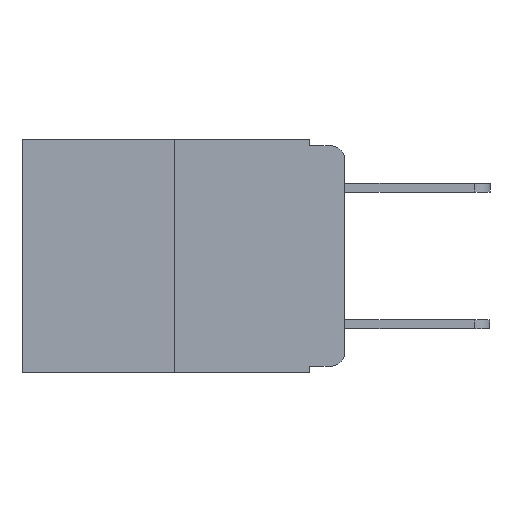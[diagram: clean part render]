
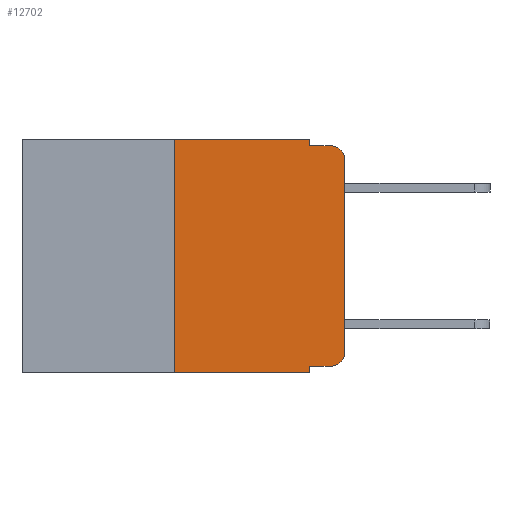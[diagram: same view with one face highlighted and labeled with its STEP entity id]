
A CAD part, left-side view. The second image highlights one B-rep face of the part: STEP entity #12702.
In plain terms, the highlighted planar face has unit normal (-1, 0, 0).
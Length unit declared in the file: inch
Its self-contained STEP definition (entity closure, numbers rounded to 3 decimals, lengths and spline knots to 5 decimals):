
#7 = CARTESIAN_POINT ( 'NONE',  ( 0., 0.051, -0.333 ) ) ;
#432 = DIRECTION ( 'NONE',  ( 0., 0., -1. ) ) ;
#626 = CARTESIAN_POINT ( 'NONE',  ( 0., 0.25, 0. ) ) ;
#860 = DIRECTION ( 'NONE',  ( 0., 0., -1. ) ) ;
#1027 = EDGE_CURVE ( 'NONE', #7281, #16380, #20398, .T. ) ;
#2823 = CARTESIAN_POINT ( 'NONE',  ( 0., 0.25, 0. ) ) ;
#3189 = VECTOR ( 'NONE', #7980, 39.37008 ) ;
#3212 = CARTESIAN_POINT ( 'NONE',  ( 0., 0., 0. ) ) ;
#3358 = ORIENTED_EDGE ( 'NONE', *, *, #3639, .T. ) ;
#3364 = CARTESIAN_POINT ( 'NONE',  ( 0., 0.051, -0.333 ) ) ;
#3558 = VERTEX_POINT ( 'NONE', #4298 ) ;
#3639 = EDGE_CURVE ( 'NONE', #3558, #7281, #15015, .T. ) ;
#3943 = EDGE_CURVE ( 'NONE', #13110, #13156, #8935, .T. ) ;
#4298 = CARTESIAN_POINT ( 'NONE',  ( 0., 0.02, -0.333 ) ) ;
#4719 = CARTESIAN_POINT ( 'NONE',  ( 0., 0.473, 0. ) ) ;
#4754 = AXIS2_PLACEMENT_3D ( 'NONE', #20390, #20478, #11328 ) ;
#5233 = ORIENTED_EDGE ( 'NONE', *, *, #3943, .F. ) ;
#5365 = DIRECTION ( 'NONE',  ( -1., 0., 0. ) ) ;
#5609 = PLANE ( 'NONE',  #8945 ) ;
#6151 = DIRECTION ( 'NONE',  ( 0., 0., 1. ) ) ;
#6529 = AXIS2_PLACEMENT_3D ( 'NONE', #15492, #5365, #17217 ) ;
#6669 = EDGE_CURVE ( 'NONE', #13178, #18244, #18235, .T. ) ;
#6810 = VECTOR ( 'NONE', #10168, 39.37008 ) ;
#7281 = VERTEX_POINT ( 'NONE', #12717 ) ;
#7354 = LINE ( 'NONE', #3364, #6810 ) ;
#7600 = ORIENTED_EDGE ( 'NONE', *, *, #8977, .F. ) ;
#7980 = DIRECTION ( 'NONE',  ( 0., -1., 0. ) ) ;
#8057 = VERTEX_POINT ( 'NONE', #10492 ) ;
#8070 = VECTOR ( 'NONE', #15999, 39.37008 ) ;
#8119 = DIRECTION ( 'NONE',  ( 0., -1., 0. ) ) ;
#8129 = VERTEX_POINT ( 'NONE', #19088 ) ;
#8935 = LINE ( 'NONE', #10293, #21849 ) ;
#8945 = AXIS2_PLACEMENT_3D ( 'NONE', #20779, #10669, #432 ) ;
#8977 = EDGE_CURVE ( 'NONE', #17702, #13110, #15774, .T. ) ;
#9217 = VECTOR ( 'NONE', #11087, 39.37008 ) ;
#9340 = CARTESIAN_POINT ( 'NONE',  ( 0., 0.051, -0.343 ) ) ;
#9372 = CARTESIAN_POINT ( 'NONE',  ( 0., 0.051, 0. ) ) ;
#9766 = ORIENTED_EDGE ( 'NONE', *, *, #1027, .T. ) ;
#9867 = DIRECTION ( 'NONE',  ( 0., -1., 0. ) ) ;
#10036 = EDGE_CURVE ( 'NONE', #8129, #17702, #12577, .T. ) ;
#10057 = CARTESIAN_POINT ( 'NONE',  ( 0., 0.051, 0. ) ) ;
#10168 = DIRECTION ( 'NONE',  ( 0., -1., 0. ) ) ;
#10293 = CARTESIAN_POINT ( 'NONE',  ( 0., 0.051, 0. ) ) ;
#10492 = CARTESIAN_POINT ( 'NONE',  ( 0., 0.02, -0.01 ) ) ;
#10669 = DIRECTION ( 'NONE',  ( 1., 0., 0. ) ) ;
#11087 = DIRECTION ( 'NONE',  ( 0., 0., -1. ) ) ;
#11268 = VECTOR ( 'NONE', #8119, 39.37008 ) ;
#11328 = DIRECTION ( 'NONE',  ( 0., 0., -1. ) ) ;
#12577 = LINE ( 'NONE', #626, #8070 ) ;
#12702 = ADVANCED_FACE ( 'NONE', ( #13420 ), #5609, .F. ) ;
#12717 = CARTESIAN_POINT ( 'NONE',  ( 0., 0., -0.313 ) ) ;
#13110 = VERTEX_POINT ( 'NONE', #10057 ) ;
#13156 = VERTEX_POINT ( 'NONE', #21993 ) ;
#13178 = VERTEX_POINT ( 'NONE', #7 ) ;
#13420 = FACE_OUTER_BOUND ( 'NONE', #16787, .T. ) ;
#14911 = CARTESIAN_POINT ( 'NONE',  ( 0., 0.473, -0.343 ) ) ;
#15015 = CIRCLE ( 'NONE', #4754, 0.02 ) ;
#15040 = ORIENTED_EDGE ( 'NONE', *, *, #20939, .F. ) ;
#15492 = CARTESIAN_POINT ( 'NONE',  ( 0., 0.02, -0.03 ) ) ;
#15774 = LINE ( 'NONE', #4719, #11268 ) ;
#15941 = ORIENTED_EDGE ( 'NONE', *, *, #21018, .T. ) ;
#15999 = DIRECTION ( 'NONE',  ( 0., 0., 1. ) ) ;
#16123 = ORIENTED_EDGE ( 'NONE', *, *, #6669, .F. ) ;
#16374 = ORIENTED_EDGE ( 'NONE', *, *, #10036, .F. ) ;
#16380 = VERTEX_POINT ( 'NONE', #20914 ) ;
#16411 = CARTESIAN_POINT ( 'NONE',  ( 0., 0.051, -0.01 ) ) ;
#16787 = EDGE_LOOP ( 'NONE', ( #9766, #18763, #15040, #5233, #7600, #16374, #15941, #16123, #17990, #3358 ) ) ;
#17217 = DIRECTION ( 'NONE',  ( 0., 0., -1. ) ) ;
#17312 = EDGE_CURVE ( 'NONE', #13178, #3558, #7354, .T. ) ;
#17702 = VERTEX_POINT ( 'NONE', #2823 ) ;
#17990 = ORIENTED_EDGE ( 'NONE', *, *, #17312, .T. ) ;
#18235 = LINE ( 'NONE', #9372, #9217 ) ;
#18244 = VERTEX_POINT ( 'NONE', #9340 ) ;
#18763 = ORIENTED_EDGE ( 'NONE', *, *, #21208, .T. ) ;
#19088 = CARTESIAN_POINT ( 'NONE',  ( 0., 0.25, -0.343 ) ) ;
#19617 = LINE ( 'NONE', #14911, #20662 ) ;
#19878 = CIRCLE ( 'NONE', #6529, 0.02 ) ;
#20390 = CARTESIAN_POINT ( 'NONE',  ( 0., 0.02, -0.313 ) ) ;
#20398 = LINE ( 'NONE', #3212, #21436 ) ;
#20478 = DIRECTION ( 'NONE',  ( -1., 0., 0. ) ) ;
#20662 = VECTOR ( 'NONE', #9867, 39.37008 ) ;
#20779 = CARTESIAN_POINT ( 'NONE',  ( 0., 0.473, 0. ) ) ;
#20914 = CARTESIAN_POINT ( 'NONE',  ( 0., 0., -0.03 ) ) ;
#20939 = EDGE_CURVE ( 'NONE', #13156, #8057, #21176, .T. ) ;
#21018 = EDGE_CURVE ( 'NONE', #8129, #18244, #19617, .T. ) ;
#21176 = LINE ( 'NONE', #16411, #3189 ) ;
#21208 = EDGE_CURVE ( 'NONE', #16380, #8057, #19878, .T. ) ;
#21436 = VECTOR ( 'NONE', #6151, 39.37008 ) ;
#21849 = VECTOR ( 'NONE', #860, 39.37008 ) ;
#21993 = CARTESIAN_POINT ( 'NONE',  ( 0., 0.051, -0.01 ) ) ;
